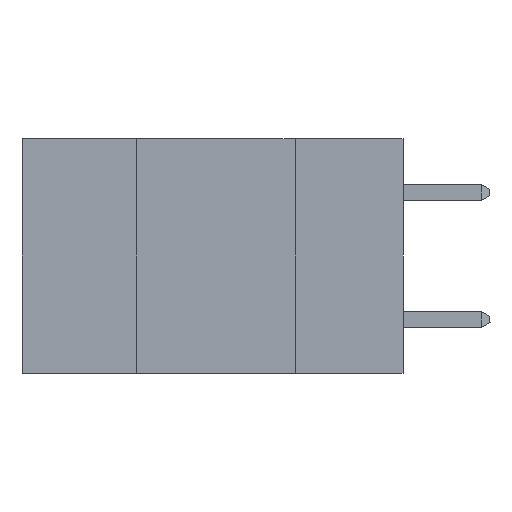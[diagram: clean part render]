
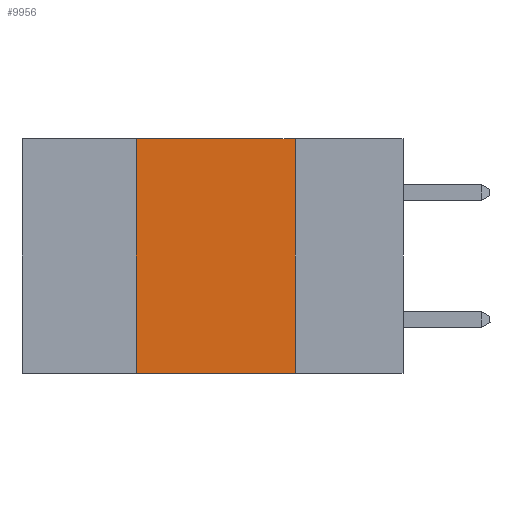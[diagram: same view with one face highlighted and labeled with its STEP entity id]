
A CAD part, left-side view. The second image highlights one B-rep face of the part: STEP entity #9956.
In plain terms, the highlighted planar face has unit normal (-1, 0, 0).
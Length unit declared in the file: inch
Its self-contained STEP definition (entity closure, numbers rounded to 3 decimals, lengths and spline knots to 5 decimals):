
#996 = LINE ( 'NONE', #3588, #9116 ) ;
#1089 = CARTESIAN_POINT ( 'NONE',  ( 0., 0.17, 0. ) ) ;
#1261 = EDGE_CURVE ( 'NONE', #6422, #15274, #2794, .T. ) ;
#1302 = PLANE ( 'NONE',  #6927 ) ;
#2190 = LINE ( 'NONE', #14864, #10737 ) ;
#2794 = LINE ( 'NONE', #13224, #19306 ) ;
#2881 = ORIENTED_EDGE ( 'NONE', *, *, #19960, .F. ) ;
#2942 = DIRECTION ( 'NONE',  ( 0., 0., -1. ) ) ;
#3128 = LINE ( 'NONE', #1089, #14867 ) ;
#3588 = CARTESIAN_POINT ( 'NONE',  ( 0., 0.42, 0. ) ) ;
#3729 = DIRECTION ( 'NONE',  ( 0., -1., 0. ) ) ;
#5236 = DIRECTION ( 'NONE',  ( 0., 0., 1. ) ) ;
#5833 = VERTEX_POINT ( 'NONE', #14943 ) ;
#6422 = VERTEX_POINT ( 'NONE', #16342 ) ;
#6927 = AXIS2_PLACEMENT_3D ( 'NONE', #10945, #12492, #2942 ) ;
#7622 = ORIENTED_EDGE ( 'NONE', *, *, #14612, .F. ) ;
#9116 = VECTOR ( 'NONE', #5236, 39.37008 ) ;
#9787 = FACE_OUTER_BOUND ( 'NONE', #15466, .T. ) ;
#9956 = ADVANCED_FACE ( 'NONE', ( #9787 ), #1302, .F. ) ;
#10734 = DIRECTION ( 'NONE',  ( 0., 0., -1. ) ) ;
#10737 = VECTOR ( 'NONE', #16492, 39.37008 ) ;
#10945 = CARTESIAN_POINT ( 'NONE',  ( 0., 0.6, 0. ) ) ;
#12492 = DIRECTION ( 'NONE',  ( 1., 0., 0. ) ) ;
#12671 = EDGE_CURVE ( 'NONE', #5833, #15274, #3128, .T. ) ;
#13158 = CARTESIAN_POINT ( 'NONE',  ( 0., 0.17, -0.37 ) ) ;
#13224 = CARTESIAN_POINT ( 'NONE',  ( 0., 0.6, -0.37 ) ) ;
#13586 = ORIENTED_EDGE ( 'NONE', *, *, #12671, .F. ) ;
#14084 = ORIENTED_EDGE ( 'NONE', *, *, #1261, .T. ) ;
#14612 = EDGE_CURVE ( 'NONE', #6422, #20530, #996, .T. ) ;
#14864 = CARTESIAN_POINT ( 'NONE',  ( 0., 0.6, 0. ) ) ;
#14867 = VECTOR ( 'NONE', #10734, 39.37008 ) ;
#14943 = CARTESIAN_POINT ( 'NONE',  ( 0., 0.17, 0. ) ) ;
#15274 = VERTEX_POINT ( 'NONE', #13158 ) ;
#15466 = EDGE_LOOP ( 'NONE', ( #13586, #2881, #7622, #14084 ) ) ;
#16342 = CARTESIAN_POINT ( 'NONE',  ( 0., 0.42, -0.37 ) ) ;
#16492 = DIRECTION ( 'NONE',  ( 0., -1., 0. ) ) ;
#19306 = VECTOR ( 'NONE', #3729, 39.37008 ) ;
#19762 = CARTESIAN_POINT ( 'NONE',  ( 0., 0.42, 0. ) ) ;
#19960 = EDGE_CURVE ( 'NONE', #20530, #5833, #2190, .T. ) ;
#20530 = VERTEX_POINT ( 'NONE', #19762 ) ;
